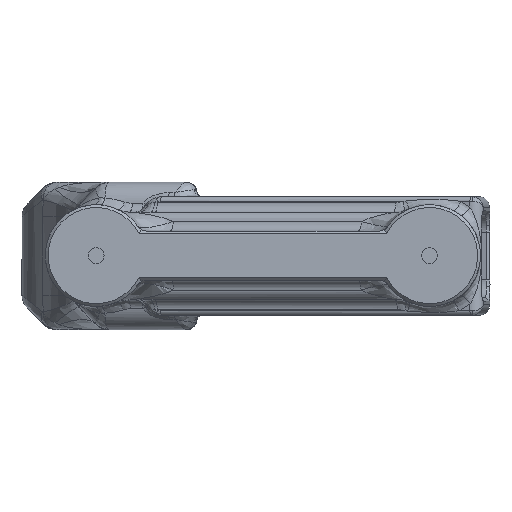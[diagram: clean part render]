
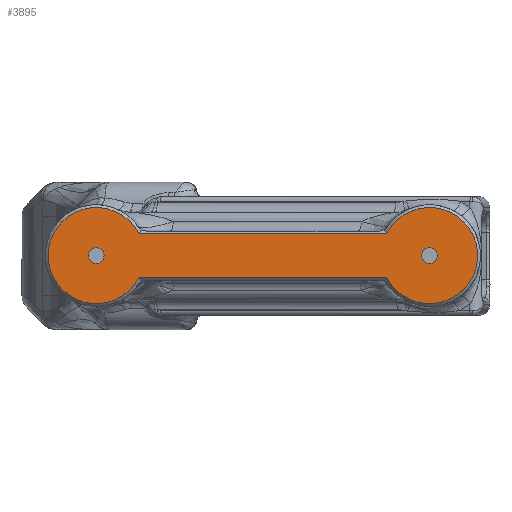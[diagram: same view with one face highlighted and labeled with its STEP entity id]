
A CAD part, left-side view. The second image highlights one B-rep face of the part: STEP entity #3895.
In plain terms, the highlighted planar face has unit normal (-1, 0, 0).
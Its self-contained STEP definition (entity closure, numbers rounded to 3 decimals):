
#212 = VERTEX_POINT ( 'NONE', #6882 ) ;
#271 = DIRECTION ( 'NONE',  ( 0., -1., 0. ) ) ;
#276 = EDGE_CURVE ( 'NONE', #7014, #11299, #7318, .T. ) ;
#538 = AXIS2_PLACEMENT_3D ( 'NONE', #17899, #9466, #2551 ) ;
#769 = DIRECTION ( 'NONE',  ( 1., 0., 0. ) ) ;
#1251 = EDGE_LOOP ( 'NONE', ( #2255, #17677, #9975, #5182 ) ) ;
#1359 = ORIENTED_EDGE ( 'NONE', *, *, #2177, .F. ) ;
#1883 = DIRECTION ( 'NONE',  ( 1., 0., 0. ) ) ;
#2177 = EDGE_CURVE ( 'NONE', #212, #212, #15097, .T. ) ;
#2255 = ORIENTED_EDGE ( 'NONE', *, *, #276, .F. ) ;
#2487 = ORIENTED_EDGE ( 'NONE', *, *, #8543, .F. ) ;
#2551 = DIRECTION ( 'NONE',  ( 0., -1., 0. ) ) ;
#2579 = AXIS2_PLACEMENT_3D ( 'NONE', #6028, #1883, #13229 ) ;
#2583 = CARTESIAN_POINT ( 'NONE',  ( -423.681, 24.664, -5.399 ) ) ;
#2650 = DIRECTION ( 'NONE',  ( 1., 0., 0. ) ) ;
#3042 = AXIS2_PLACEMENT_3D ( 'NONE', #7840, #769, #13197 ) ;
#3537 = CARTESIAN_POINT ( 'NONE',  ( -423.681, 12.448, 7.001 ) ) ;
#3592 = CARTESIAN_POINT ( 'NONE',  ( -423.681, 12.447, -5.399 ) ) ;
#3766 = DIRECTION ( 'NONE',  ( 0., 0., -1. ) ) ;
#3895 = ADVANCED_FACE ( 'NONE', ( #11550, #17034, #10443 ), #6095, .F. ) ;
#4407 = VECTOR ( 'NONE', #12522, 1000. ) ;
#4982 = CARTESIAN_POINT ( 'NONE',  ( -423.681, -70.336, 0.8 ) ) ;
#5032 = AXIS2_PLACEMENT_3D ( 'NONE', #4982, #2650, #3766 ) ;
#5182 = ORIENTED_EDGE ( 'NONE', *, *, #8388, .F. ) ;
#5743 = DIRECTION ( 'NONE',  ( 0., 1., 0. ) ) ;
#5746 = VERTEX_POINT ( 'NONE', #10949 ) ;
#6028 = CARTESIAN_POINT ( 'NONE',  ( -423.681, 24.664, 0.8 ) ) ;
#6095 = PLANE ( 'NONE',  #2579 ) ;
#6640 = CIRCLE ( 'NONE', #12331, 2.25 ) ;
#6680 = VERTEX_POINT ( 'NONE', #3537 ) ;
#6882 = CARTESIAN_POINT ( 'NONE',  ( -423.681, 22.414, 0.8 ) ) ;
#7014 = VERTEX_POINT ( 'NONE', #14638 ) ;
#7318 = CIRCLE ( 'NONE', #5032, 13.7 ) ;
#7334 = CARTESIAN_POINT ( 'NONE',  ( -423.681, -22.321, 7.001 ) ) ;
#7840 = CARTESIAN_POINT ( 'NONE',  ( -423.681, 24.664, 0.8 ) ) ;
#8116 = EDGE_LOOP ( 'NONE', ( #1359 ) ) ;
#8388 = EDGE_CURVE ( 'NONE', #11299, #11348, #10818, .T. ) ;
#8543 = EDGE_CURVE ( 'NONE', #5746, #5746, #6640, .T. ) ;
#8762 = CARTESIAN_POINT ( 'NONE',  ( -423.681, -70.336, 0.8 ) ) ;
#9466 = DIRECTION ( 'NONE',  ( -1., 0., 0. ) ) ;
#9523 = LINE ( 'NONE', #7334, #14173 ) ;
#9975 = ORIENTED_EDGE ( 'NONE', *, *, #13837, .F. ) ;
#10443 = FACE_OUTER_BOUND ( 'NONE', #1251, .T. ) ;
#10818 = LINE ( 'NONE', #2583, #4407 ) ;
#10949 = CARTESIAN_POINT ( 'NONE',  ( -423.681, -68.086, 0.8 ) ) ;
#11299 = VERTEX_POINT ( 'NONE', #11574 ) ;
#11348 = VERTEX_POINT ( 'NONE', #3592 ) ;
#11550 = FACE_BOUND ( 'NONE', #12075, .T. ) ;
#11574 = CARTESIAN_POINT ( 'NONE',  ( -423.681, -58.119, -5.399 ) ) ;
#12075 = EDGE_LOOP ( 'NONE', ( #2487 ) ) ;
#12331 = AXIS2_PLACEMENT_3D ( 'NONE', #8762, #15537, #5743 ) ;
#12522 = DIRECTION ( 'NONE',  ( 0., 1., 0. ) ) ;
#13197 = DIRECTION ( 'NONE',  ( 0., 0., -1. ) ) ;
#13229 = DIRECTION ( 'NONE',  ( 0., 1., 0. ) ) ;
#13837 = EDGE_CURVE ( 'NONE', #11348, #6680, #16374, .T. ) ;
#14173 = VECTOR ( 'NONE', #271, 1000. ) ;
#14638 = CARTESIAN_POINT ( 'NONE',  ( -423.681, -58.119, 7.001 ) ) ;
#15097 = CIRCLE ( 'NONE', #538, 2.25 ) ;
#15537 = DIRECTION ( 'NONE',  ( -1., 0., 0. ) ) ;
#16221 = EDGE_CURVE ( 'NONE', #6680, #7014, #9523, .T. ) ;
#16374 = CIRCLE ( 'NONE', #3042, 13.7 ) ;
#17034 = FACE_BOUND ( 'NONE', #8116, .T. ) ;
#17677 = ORIENTED_EDGE ( 'NONE', *, *, #16221, .F. ) ;
#17899 = CARTESIAN_POINT ( 'NONE',  ( -423.681, 24.664, 0.8 ) ) ;
